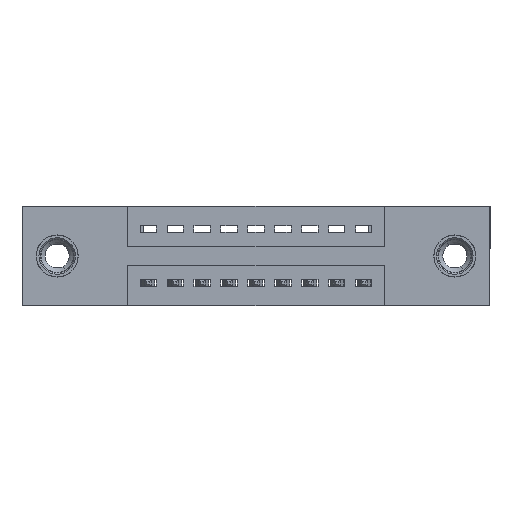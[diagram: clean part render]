
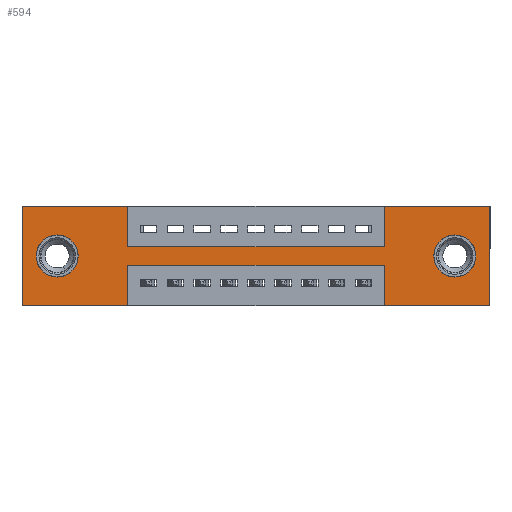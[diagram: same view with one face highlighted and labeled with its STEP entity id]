
A CAD part, front view. The second image highlights one B-rep face of the part: STEP entity #594.
In plain terms, the highlighted planar face has unit normal (0, -1, 0).
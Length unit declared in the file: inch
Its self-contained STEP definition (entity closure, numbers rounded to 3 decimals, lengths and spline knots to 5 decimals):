
#32 = ORIENTED_EDGE ( 'NONE', *, *, #3528, .T. ) ;
#125 = ORIENTED_EDGE ( 'NONE', *, *, #3014, .F. ) ;
#140 = DIRECTION ( 'NONE',  ( 1., 0., 0. ) ) ;
#465 = VECTOR ( 'NONE', #10986, 39.37008 ) ;
#488 = FACE_OUTER_BOUND ( 'NONE', #1884, .T. ) ;
#594 = ADVANCED_FACE ( 'NONE', ( #5849, #14549, #488 ), #2649, .T. ) ;
#807 = VECTOR ( 'NONE', #2034, 39.37008 ) ;
#1200 = VERTEX_POINT ( 'NONE', #12603 ) ;
#1279 = DIRECTION ( 'NONE',  ( 0., 0., -1. ) ) ;
#1413 = DIRECTION ( 'NONE',  ( 0., 0., 1. ) ) ;
#1565 = EDGE_CURVE ( 'NONE', #1669, #7534, #5265, .T. ) ;
#1569 = ORIENTED_EDGE ( 'NONE', *, *, #13009, .F. ) ;
#1582 = ORIENTED_EDGE ( 'NONE', *, *, #14188, .F. ) ;
#1664 = VERTEX_POINT ( 'NONE', #16017 ) ;
#1669 = VERTEX_POINT ( 'NONE', #6069 ) ;
#1785 = EDGE_CURVE ( 'NONE', #13274, #1669, #11618, .T. ) ;
#1884 = EDGE_LOOP ( 'NONE', ( #4859, #125, #1582, #1569, #14638, #9659, #9454, #12512, #15562, #5330, #11812, #8376 ) ) ;
#1921 = AXIS2_PLACEMENT_3D ( 'NONE', #3464, #13784, #3954 ) ;
#2034 = DIRECTION ( 'NONE',  ( -1., 0., 0. ) ) ;
#2178 = CARTESIAN_POINT ( 'NONE',  ( 0.13, 0., -0.185 ) ) ;
#2283 = EDGE_LOOP ( 'NONE', ( #32, #5139 ) ) ;
#2340 = CARTESIAN_POINT ( 'NONE',  ( 0., 0., 0. ) ) ;
#2360 = CARTESIAN_POINT ( 'NONE',  ( 0., 0., 0. ) ) ;
#2411 = VECTOR ( 'NONE', #4109, 39.37008 ) ;
#2415 = DIRECTION ( 'NONE',  ( 0., 0., 1. ) ) ;
#2476 = VERTEX_POINT ( 'NONE', #9992 ) ;
#2563 = CARTESIAN_POINT ( 'NONE',  ( 1.605, 0., -0.263 ) ) ;
#2590 = CARTESIAN_POINT ( 'NONE',  ( 0., 0., -0.37 ) ) ;
#2649 = PLANE ( 'NONE',  #6122 ) ;
#3014 = EDGE_CURVE ( 'NONE', #6014, #13274, #14472, .T. ) ;
#3022 = VECTOR ( 'NONE', #6836, 39.37008 ) ;
#3399 = EDGE_CURVE ( 'NONE', #11946, #6065, #6143, .T. ) ;
#3451 = VECTOR ( 'NONE', #5994, 39.37008 ) ;
#3464 = CARTESIAN_POINT ( 'NONE',  ( 1.605, 0., -0.185 ) ) ;
#3488 = DIRECTION ( 'NONE',  ( -1., 0., 0. ) ) ;
#3528 = EDGE_CURVE ( 'NONE', #6065, #11946, #15320, .T. ) ;
#3736 = CARTESIAN_POINT ( 'NONE',  ( 0.13, 0., -0.185 ) ) ;
#3949 = VECTOR ( 'NONE', #140, 39.37008 ) ;
#3954 = DIRECTION ( 'NONE',  ( 0., 0., -1. ) ) ;
#4028 = VECTOR ( 'NONE', #11180, 39.37008 ) ;
#4068 = VECTOR ( 'NONE', #1279, 39.37008 ) ;
#4109 = DIRECTION ( 'NONE',  ( 0., 0., 1. ) ) ;
#4134 = CARTESIAN_POINT ( 'NONE',  ( 0.13, 0., -0.107 ) ) ;
#4755 = CARTESIAN_POINT ( 'NONE',  ( 0.3925, 0., 0. ) ) ;
#4859 = ORIENTED_EDGE ( 'NONE', *, *, #1785, .F. ) ;
#4984 = DIRECTION ( 'NONE',  ( 0., 1., 0. ) ) ;
#5139 = ORIENTED_EDGE ( 'NONE', *, *, #3399, .T. ) ;
#5265 = LINE ( 'NONE', #8196, #807 ) ;
#5330 = ORIENTED_EDGE ( 'NONE', *, *, #8187, .F. ) ;
#5458 = CARTESIAN_POINT ( 'NONE',  ( 1.605, 0., -0.185 ) ) ;
#5591 = VECTOR ( 'NONE', #7971, 39.37008 ) ;
#5849 = FACE_BOUND ( 'NONE', #2283, .T. ) ;
#5923 = VERTEX_POINT ( 'NONE', #4134 ) ;
#5994 = DIRECTION ( 'NONE',  ( 1., 0., 0. ) ) ;
#6014 = VERTEX_POINT ( 'NONE', #11668 ) ;
#6042 = LINE ( 'NONE', #2340, #15533 ) ;
#6065 = VERTEX_POINT ( 'NONE', #13658 ) ;
#6069 = CARTESIAN_POINT ( 'NONE',  ( 0.3925, 0., -0.37 ) ) ;
#6122 = AXIS2_PLACEMENT_3D ( 'NONE', #2590, #12455, #12621 ) ;
#6143 = CIRCLE ( 'NONE', #1921, 0.078 ) ;
#6248 = LINE ( 'NONE', #11477, #2411 ) ;
#6634 = LINE ( 'NONE', #4755, #465 ) ;
#6836 = DIRECTION ( 'NONE',  ( 1., 0., 0. ) ) ;
#7308 = EDGE_CURVE ( 'NONE', #1664, #5923, #9616, .T. ) ;
#7534 = VERTEX_POINT ( 'NONE', #15949 ) ;
#7693 = LINE ( 'NONE', #14929, #4028 ) ;
#7865 = EDGE_LOOP ( 'NONE', ( #10971, #15343 ) ) ;
#7924 = DIRECTION ( 'NONE',  ( 0., 0., -1. ) ) ;
#7958 = CARTESIAN_POINT ( 'NONE',  ( 0.3925, 0., -0.22 ) ) ;
#7971 = DIRECTION ( 'NONE',  ( -1., 0., 0. ) ) ;
#8187 = EDGE_CURVE ( 'NONE', #13045, #16009, #12861, .T. ) ;
#8196 = CARTESIAN_POINT ( 'NONE',  ( 0., 0., -0.37 ) ) ;
#8376 = ORIENTED_EDGE ( 'NONE', *, *, #1565, .F. ) ;
#8391 = DIRECTION ( 'NONE',  ( 0., 1., 0. ) ) ;
#8762 = CARTESIAN_POINT ( 'NONE',  ( 0.3925, 0., -0.15 ) ) ;
#8770 = LINE ( 'NONE', #8762, #3949 ) ;
#9238 = CARTESIAN_POINT ( 'NONE',  ( 1.3425, 0., -0.37 ) ) ;
#9454 = ORIENTED_EDGE ( 'NONE', *, *, #12013, .F. ) ;
#9509 = VECTOR ( 'NONE', #10298, 39.37008 ) ;
#9616 = CIRCLE ( 'NONE', #15628, 0.078 ) ;
#9659 = ORIENTED_EDGE ( 'NONE', *, *, #11786, .F. ) ;
#9992 = CARTESIAN_POINT ( 'NONE',  ( 1.735, 0., -0.37 ) ) ;
#10298 = DIRECTION ( 'NONE',  ( 0., 0., -1. ) ) ;
#10406 = CARTESIAN_POINT ( 'NONE',  ( 0.3925, 0., -0.15 ) ) ;
#10463 = VERTEX_POINT ( 'NONE', #11968 ) ;
#10904 = CARTESIAN_POINT ( 'NONE',  ( 0., 0., -0.37 ) ) ;
#10971 = ORIENTED_EDGE ( 'NONE', *, *, #12953, .T. ) ;
#10986 = DIRECTION ( 'NONE',  ( 0., 0., -1. ) ) ;
#11010 = VERTEX_POINT ( 'NONE', #11959 ) ;
#11180 = DIRECTION ( 'NONE',  ( 0., 0., 1. ) ) ;
#11329 = EDGE_CURVE ( 'NONE', #1200, #2476, #15639, .T. ) ;
#11477 = CARTESIAN_POINT ( 'NONE',  ( 1.3425, 0., -0.37 ) ) ;
#11487 = CARTESIAN_POINT ( 'NONE',  ( 0.3925, 0., -0.22 ) ) ;
#11618 = LINE ( 'NONE', #13989, #9509 ) ;
#11668 = CARTESIAN_POINT ( 'NONE',  ( 1.3425, 0., -0.22 ) ) ;
#11710 = CIRCLE ( 'NONE', #15881, 0.078 ) ;
#11786 = EDGE_CURVE ( 'NONE', #10463, #1200, #12332, .T. ) ;
#11812 = ORIENTED_EDGE ( 'NONE', *, *, #14495, .F. ) ;
#11946 = VERTEX_POINT ( 'NONE', #2563 ) ;
#11959 = CARTESIAN_POINT ( 'NONE',  ( 1.3425, 0., -0.15 ) ) ;
#11968 = CARTESIAN_POINT ( 'NONE',  ( 1.3425, 0., 0. ) ) ;
#12013 = EDGE_CURVE ( 'NONE', #11010, #10463, #7693, .T. ) ;
#12097 = DIRECTION ( 'NONE',  ( 0., 0., 1. ) ) ;
#12332 = LINE ( 'NONE', #13507, #3451 ) ;
#12455 = DIRECTION ( 'NONE',  ( 0., -1., 0. ) ) ;
#12512 = ORIENTED_EDGE ( 'NONE', *, *, #14658, .F. ) ;
#12603 = CARTESIAN_POINT ( 'NONE',  ( 1.735, 0., 0. ) ) ;
#12621 = DIRECTION ( 'NONE',  ( 0., 0., -1. ) ) ;
#12662 = VERTEX_POINT ( 'NONE', #9238 ) ;
#12776 = VERTEX_POINT ( 'NONE', #10406 ) ;
#12861 = LINE ( 'NONE', #14339, #3022 ) ;
#12953 = EDGE_CURVE ( 'NONE', #5923, #1664, #11710, .T. ) ;
#13009 = EDGE_CURVE ( 'NONE', #2476, #12662, #13442, .T. ) ;
#13045 = VERTEX_POINT ( 'NONE', #2360 ) ;
#13274 = VERTEX_POINT ( 'NONE', #7958 ) ;
#13295 = AXIS2_PLACEMENT_3D ( 'NONE', #5458, #14106, #7924 ) ;
#13442 = LINE ( 'NONE', #10904, #14398 ) ;
#13507 = CARTESIAN_POINT ( 'NONE',  ( 0., 0., 0. ) ) ;
#13658 = CARTESIAN_POINT ( 'NONE',  ( 1.605, 0., -0.107 ) ) ;
#13784 = DIRECTION ( 'NONE',  ( 0., 1., 0. ) ) ;
#13989 = CARTESIAN_POINT ( 'NONE',  ( 0.3925, 0., -0.37 ) ) ;
#14106 = DIRECTION ( 'NONE',  ( 0., 1., 0. ) ) ;
#14188 = EDGE_CURVE ( 'NONE', #12662, #6014, #6248, .T. ) ;
#14261 = CARTESIAN_POINT ( 'NONE',  ( 0.3925, 0., 0. ) ) ;
#14339 = CARTESIAN_POINT ( 'NONE',  ( 0., 0., 0. ) ) ;
#14398 = VECTOR ( 'NONE', #3488, 39.37008 ) ;
#14472 = LINE ( 'NONE', #11487, #5591 ) ;
#14495 = EDGE_CURVE ( 'NONE', #7534, #13045, #6042, .T. ) ;
#14549 = FACE_BOUND ( 'NONE', #7865, .T. ) ;
#14638 = ORIENTED_EDGE ( 'NONE', *, *, #11329, .F. ) ;
#14658 = EDGE_CURVE ( 'NONE', #12776, #11010, #8770, .T. ) ;
#14833 = CARTESIAN_POINT ( 'NONE',  ( 1.735, 0., 0. ) ) ;
#14929 = CARTESIAN_POINT ( 'NONE',  ( 1.3425, 0., 0. ) ) ;
#15200 = EDGE_CURVE ( 'NONE', #16009, #12776, #6634, .T. ) ;
#15320 = CIRCLE ( 'NONE', #13295, 0.078 ) ;
#15343 = ORIENTED_EDGE ( 'NONE', *, *, #7308, .T. ) ;
#15533 = VECTOR ( 'NONE', #12097, 39.37008 ) ;
#15562 = ORIENTED_EDGE ( 'NONE', *, *, #15200, .F. ) ;
#15628 = AXIS2_PLACEMENT_3D ( 'NONE', #3736, #4984, #1413 ) ;
#15639 = LINE ( 'NONE', #14833, #4068 ) ;
#15881 = AXIS2_PLACEMENT_3D ( 'NONE', #2178, #8391, #2415 ) ;
#15949 = CARTESIAN_POINT ( 'NONE',  ( 0., 0., -0.37 ) ) ;
#16009 = VERTEX_POINT ( 'NONE', #14261 ) ;
#16017 = CARTESIAN_POINT ( 'NONE',  ( 0.13, 0., -0.263 ) ) ;
